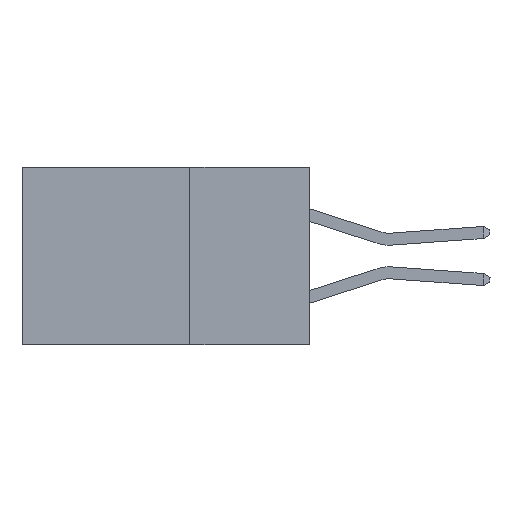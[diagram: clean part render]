
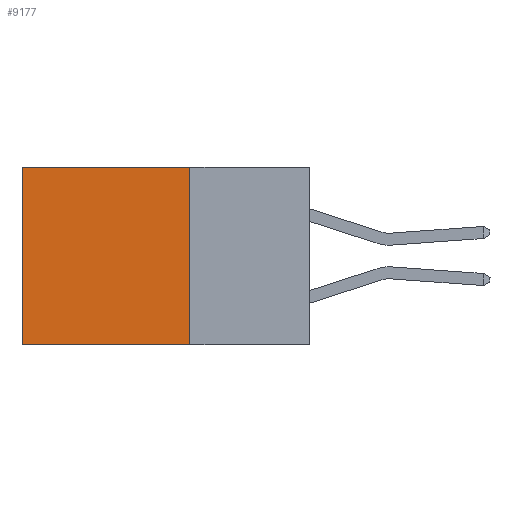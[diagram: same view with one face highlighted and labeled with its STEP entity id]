
A CAD part, left-side view. The second image highlights one B-rep face of the part: STEP entity #9177.
In plain terms, the highlighted planar face has unit normal (-1, 0, 0).
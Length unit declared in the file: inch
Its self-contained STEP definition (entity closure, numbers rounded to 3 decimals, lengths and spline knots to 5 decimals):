
#397 = CARTESIAN_POINT ( 'NONE',  ( 0.2615, 0.25, -0.37 ) ) ;
#807 = PLANE ( 'NONE',  #8599 ) ;
#1530 = VERTEX_POINT ( 'NONE', #1772 ) ;
#1772 = CARTESIAN_POINT ( 'NONE',  ( 0.2615, 0.6, 0. ) ) ;
#2056 = ORIENTED_EDGE ( 'NONE', *, *, #6248, .F. ) ;
#2128 = ORIENTED_EDGE ( 'NONE', *, *, #16119, .F. ) ;
#2746 = DIRECTION ( 'NONE',  ( 1., 0., 0. ) ) ;
#3122 = LINE ( 'NONE', #21151, #12877 ) ;
#4619 = EDGE_CURVE ( 'NONE', #1530, #13613, #14498, .T. ) ;
#5341 = VECTOR ( 'NONE', #11396, 39.37008 ) ;
#6248 = EDGE_CURVE ( 'NONE', #20411, #13613, #3122, .T. ) ;
#6858 = VECTOR ( 'NONE', #15425, 39.37008 ) ;
#8599 = AXIS2_PLACEMENT_3D ( 'NONE', #12441, #2746, #16325 ) ;
#9177 = ADVANCED_FACE ( 'NONE', ( #11165 ), #807, .F. ) ;
#10076 = DIRECTION ( 'NONE',  ( 0., 0., -1. ) ) ;
#10473 = CARTESIAN_POINT ( 'NONE',  ( 0.2615, 0.6, -0.37 ) ) ;
#11165 = FACE_OUTER_BOUND ( 'NONE', #15509, .T. ) ;
#11396 = DIRECTION ( 'NONE',  ( 0., 0., -1. ) ) ;
#11425 = CARTESIAN_POINT ( 'NONE',  ( 0.2615, 0.6, -0.37 ) ) ;
#12441 = CARTESIAN_POINT ( 'NONE',  ( 0.2615, 0.25, -0.37 ) ) ;
#12607 = VECTOR ( 'NONE', #10076, 39.37008 ) ;
#12877 = VECTOR ( 'NONE', #21232, 39.37008 ) ;
#13219 = LINE ( 'NONE', #397, #12607 ) ;
#13488 = CARTESIAN_POINT ( 'NONE',  ( 0.2615, 0.25, 0. ) ) ;
#13613 = VERTEX_POINT ( 'NONE', #10473 ) ;
#14498 = LINE ( 'NONE', #11425, #5341 ) ;
#15238 = EDGE_CURVE ( 'NONE', #20552, #1530, #22301, .T. ) ;
#15425 = DIRECTION ( 'NONE',  ( 0., 1., 0. ) ) ;
#15509 = EDGE_LOOP ( 'NONE', ( #20079, #2056, #2128, #19598 ) ) ;
#16119 = EDGE_CURVE ( 'NONE', #20552, #20411, #13219, .T. ) ;
#16325 = DIRECTION ( 'NONE',  ( 0., 0., -1. ) ) ;
#19598 = ORIENTED_EDGE ( 'NONE', *, *, #15238, .T. ) ;
#20079 = ORIENTED_EDGE ( 'NONE', *, *, #4619, .T. ) ;
#20271 = CARTESIAN_POINT ( 'NONE',  ( 0.2615, 0.25, 0. ) ) ;
#20411 = VERTEX_POINT ( 'NONE', #21782 ) ;
#20552 = VERTEX_POINT ( 'NONE', #20271 ) ;
#21151 = CARTESIAN_POINT ( 'NONE',  ( 0.2615, 0.25, -0.37 ) ) ;
#21232 = DIRECTION ( 'NONE',  ( 0., 1., 0. ) ) ;
#21782 = CARTESIAN_POINT ( 'NONE',  ( 0.2615, 0.25, -0.37 ) ) ;
#22301 = LINE ( 'NONE', #13488, #6858 ) ;
